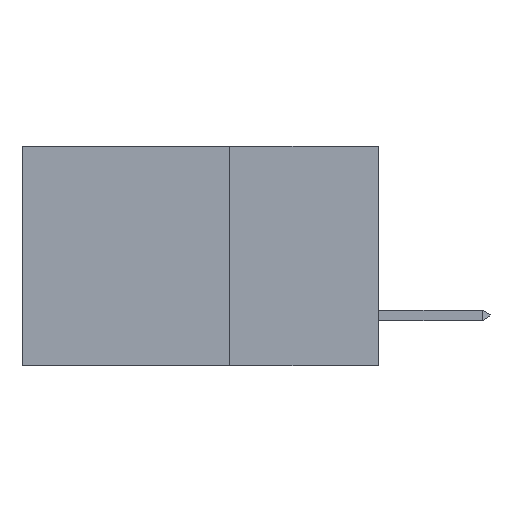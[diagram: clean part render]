
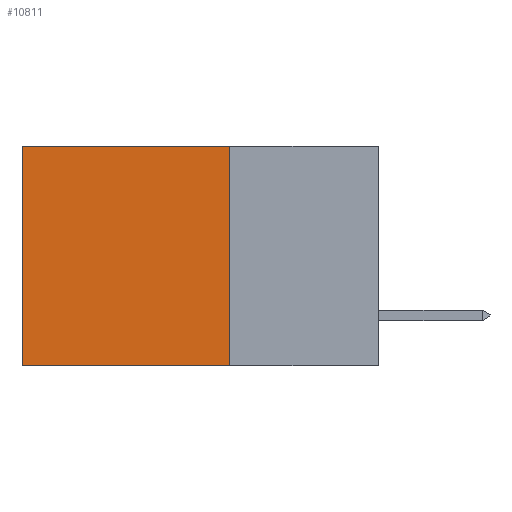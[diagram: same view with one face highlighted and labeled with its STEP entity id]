
A CAD part, left-side view. The second image highlights one B-rep face of the part: STEP entity #10811.
In plain terms, the highlighted planar face has unit normal (-1, 0, 0).
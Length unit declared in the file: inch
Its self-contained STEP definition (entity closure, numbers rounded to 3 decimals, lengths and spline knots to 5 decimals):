
#606 = VECTOR ( 'NONE', #15527, 39.37008 ) ;
#1374 = DIRECTION ( 'NONE',  ( 0., 0., -1. ) ) ;
#2842 = FACE_OUTER_BOUND ( 'NONE', #6244, .T. ) ;
#3062 = LINE ( 'NONE', #3464, #15168 ) ;
#3464 = CARTESIAN_POINT ( 'NONE',  ( 0.298, 0.25, 0. ) ) ;
#4069 = EDGE_CURVE ( 'NONE', #25145, #11959, #20372, .T. ) ;
#6244 = EDGE_LOOP ( 'NONE', ( #6370, #28569, #18487, #6897 ) ) ;
#6370 = ORIENTED_EDGE ( 'NONE', *, *, #4069, .T. ) ;
#6409 = EDGE_CURVE ( 'NONE', #24149, #11959, #7453, .T. ) ;
#6492 = DIRECTION ( 'NONE',  ( 0., 0., -1. ) ) ;
#6897 = ORIENTED_EDGE ( 'NONE', *, *, #16989, .T. ) ;
#7453 = LINE ( 'NONE', #11176, #606 ) ;
#7613 = DIRECTION ( 'NONE',  ( 0., 0., -1. ) ) ;
#8404 = CARTESIAN_POINT ( 'NONE',  ( 0.298, 0.6, 0. ) ) ;
#8571 = DIRECTION ( 'NONE',  ( 1., 0., 0. ) ) ;
#8665 = VECTOR ( 'NONE', #7613, 39.37008 ) ;
#9210 = EDGE_CURVE ( 'NONE', #10785, #24149, #17892, .T. ) ;
#10785 = VERTEX_POINT ( 'NONE', #23848 ) ;
#10811 = ADVANCED_FACE ( 'NONE', ( #2842 ), #28722, .F. ) ;
#11176 = CARTESIAN_POINT ( 'NONE',  ( 0.298, 0.25, -0.37 ) ) ;
#11959 = VERTEX_POINT ( 'NONE', #25318 ) ;
#13539 = CARTESIAN_POINT ( 'NONE',  ( 0.298, 0.25, 0. ) ) ;
#15168 = VECTOR ( 'NONE', #26303, 39.37008 ) ;
#15527 = DIRECTION ( 'NONE',  ( 0., 1., 0. ) ) ;
#16989 = EDGE_CURVE ( 'NONE', #10785, #25145, #3062, .T. ) ;
#17874 = VECTOR ( 'NONE', #1374, 39.37008 ) ;
#17892 = LINE ( 'NONE', #13539, #8665 ) ;
#18487 = ORIENTED_EDGE ( 'NONE', *, *, #9210, .F. ) ;
#19970 = AXIS2_PLACEMENT_3D ( 'NONE', #22187, #8571, #6492 ) ;
#20372 = LINE ( 'NONE', #8404, #17874 ) ;
#22187 = CARTESIAN_POINT ( 'NONE',  ( 0.298, 0.25, 0. ) ) ;
#23848 = CARTESIAN_POINT ( 'NONE',  ( 0.298, 0.25, 0. ) ) ;
#24149 = VERTEX_POINT ( 'NONE', #26777 ) ;
#25145 = VERTEX_POINT ( 'NONE', #28948 ) ;
#25318 = CARTESIAN_POINT ( 'NONE',  ( 0.298, 0.6, -0.37 ) ) ;
#26303 = DIRECTION ( 'NONE',  ( 0., 1., 0. ) ) ;
#26777 = CARTESIAN_POINT ( 'NONE',  ( 0.298, 0.25, -0.37 ) ) ;
#28569 = ORIENTED_EDGE ( 'NONE', *, *, #6409, .F. ) ;
#28722 = PLANE ( 'NONE',  #19970 ) ;
#28948 = CARTESIAN_POINT ( 'NONE',  ( 0.298, 0.6, 0. ) ) ;
